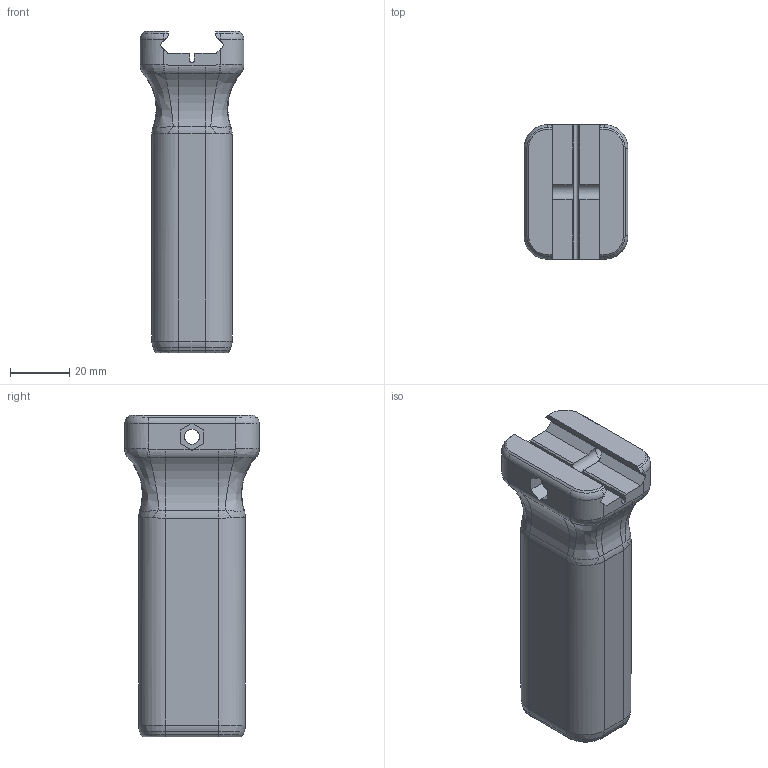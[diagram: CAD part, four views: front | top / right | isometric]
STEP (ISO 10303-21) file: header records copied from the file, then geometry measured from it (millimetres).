
FILE_DESCRIPTION(/* description */ (''),/* implementation_level */ '2;1');
FILE_NAME(/* name */ 'Basic Model.step',/* time_stamp */ '2021-05-21T12:31:15-04:00',/* author */ (''),/* organization */ (''),/* preprocessor_version */ 'ST-DEVELOPER v18.1',/* originating_system */ 'Autodesk Translation Framework v10.6.0.1341',/* authorisation */ '');
FILE_SCHEMA (('AUTOMOTIVE_DESIGN { 1 0 10303 214 3 1 1 }'));
Length unit declared in the file: millimetre
Products named in the file (1): Basic Model
Bounding box: 35 x 45.3 x 108.12 mm (x, y, z)
Volume: 56790.6 mm3; surface area: 23412.1 mm2
Topology: 1 solids, 1 shells, 267 faces, 623 edges, 358 vertices
Faces by surface type: bspline 84, cylinder 80, plane 71, torus 20, cone 12
Full cylindrical faces by diameter (mm): 5.1 x2, 8.75 x1, 11.5 x1, 13 x1
Entity records: 9490 total; most frequent: CARTESIAN_POINT 3766, ORIENTED_EDGE 1238, DIRECTION 1099, EDGE_CURVE 619, AXIS2_PLACEMENT_3D 432, VERTEX_POINT 358, EDGE_LOOP 275, FACE_OUTER_BOUND 267
